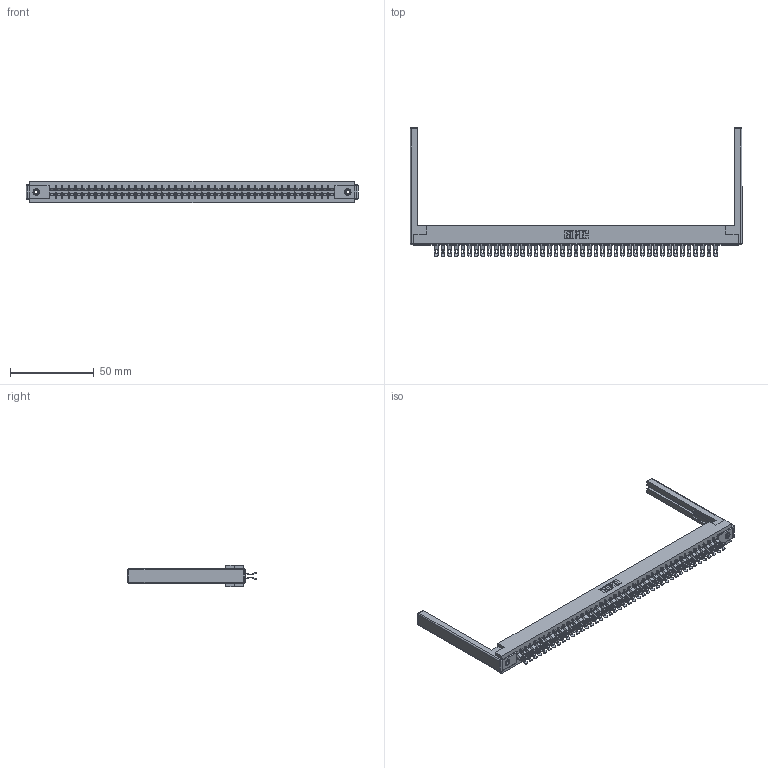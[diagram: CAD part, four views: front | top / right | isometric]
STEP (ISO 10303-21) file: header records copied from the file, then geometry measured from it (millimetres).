
FILE_DESCRIPTION (( 'STEP AP203' ), '1' );
FILE_NAME ('305-086-555-568.STEP', '2019-09-10T13:04:32', ( '' ), ( '' ), 'SwSTEP 2.0', 'SolidWorks 2016', '' );
FILE_SCHEMA (( 'CONFIG_CONTROL_DESIGN' ));
Length unit declared in the file: inch
Products named in the file (5): 307-220-068; 305 Part_.156 Dia; 305-086-555-568; 305-290-001_555; 345-250-001_345-250-001-102
Assembly tree (91 placements, depth 2):
  305-086-555-568
    305 Part_.156 Dia
    305-290-001_555  x86
    345-250-001_345-250-001-102  x2
    307-220-068  x2
Bounding box: 197.82 x 76.71 x 12.7 mm (x, y, z)
Volume: 24692.5 mm3; surface area: 32393.2 mm2
Topology: 91 solids, 91 shells, 5946 faces, 17691 edges, 11542 vertices
Faces by surface type: plane 2908, cylinder 2842, sphere 180, cone 12, torus 4
Entity records: 49819 total; most frequent: CARTESIAN_POINT 8234, ORIENTED_EDGE 8156, DIRECTION 7978, EDGE_CURVE 4078, VECTOR 3270, LINE 3270, VERTEX_POINT 2594, AXIS2_PLACEMENT_3D 2354
